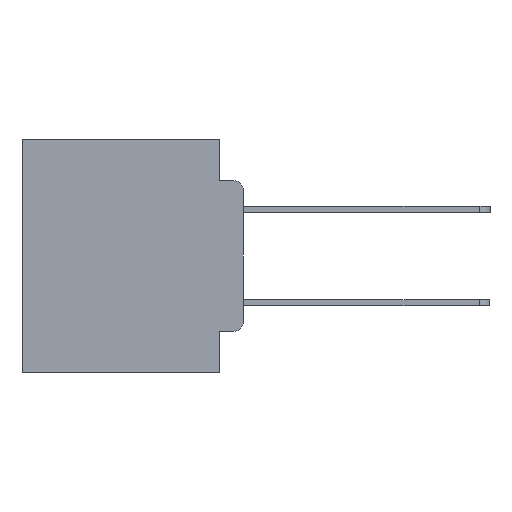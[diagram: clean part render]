
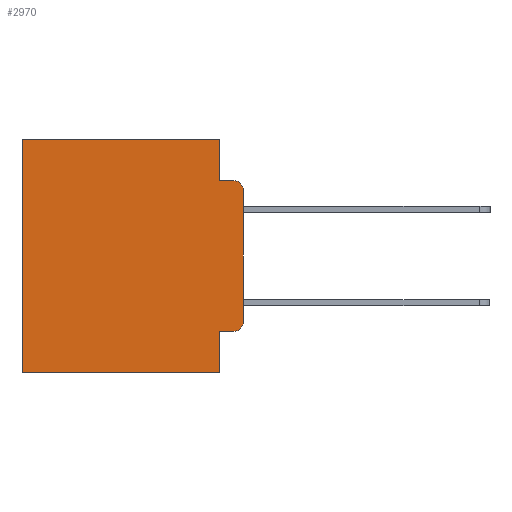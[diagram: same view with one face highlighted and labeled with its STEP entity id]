
A CAD part, left-side view. The second image highlights one B-rep face of the part: STEP entity #2970.
In plain terms, the highlighted planar face has unit normal (-1, 0, 0).
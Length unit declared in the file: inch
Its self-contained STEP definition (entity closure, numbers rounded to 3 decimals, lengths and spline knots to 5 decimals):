
#511 = EDGE_CURVE ( 'NONE', #17924, #20325, #26885, .T. ) ;
#786 = DIRECTION ( 'NONE',  ( 1., 0., 0. ) ) ;
#950 = EDGE_CURVE ( 'NONE', #10034, #12043, #11070, .T. ) ;
#1127 = DIRECTION ( 'NONE',  ( 0., 0., -1. ) ) ;
#1162 = CARTESIAN_POINT ( 'NONE',  ( 0.298, 0.051, -0.5 ) ) ;
#1786 = DIRECTION ( 'NONE',  ( 0., 0., -1. ) ) ;
#1940 = CARTESIAN_POINT ( 'NONE',  ( 0.298, 0.473, 0. ) ) ;
#2078 = CARTESIAN_POINT ( 'NONE',  ( 0.298, 0., 0. ) ) ;
#2630 = ORIENTED_EDGE ( 'NONE', *, *, #7078, .F. ) ;
#2756 = CARTESIAN_POINT ( 'NONE',  ( 0.298, 0.02, -0.0885 ) ) ;
#2970 = ADVANCED_FACE ( 'NONE', ( #5339 ), #6437, .F. ) ;
#3046 = VERTEX_POINT ( 'NONE', #18822 ) ;
#4294 = VERTEX_POINT ( 'NONE', #19255 ) ;
#4443 = DIRECTION ( 'NONE',  ( -1., 0., 0. ) ) ;
#4648 = DIRECTION ( 'NONE',  ( 0., -1., 0. ) ) ;
#4677 = EDGE_CURVE ( 'NONE', #3046, #8302, #20778, .T. ) ;
#4717 = ORIENTED_EDGE ( 'NONE', *, *, #4677, .F. ) ;
#4980 = CIRCLE ( 'NONE', #23388, 0.02 ) ;
#5144 = DIRECTION ( 'NONE',  ( 0., 0., -1. ) ) ;
#5167 = CARTESIAN_POINT ( 'NONE',  ( 0.298, 0.051, -0.4115 ) ) ;
#5240 = ORIENTED_EDGE ( 'NONE', *, *, #21757, .T. ) ;
#5339 = FACE_OUTER_BOUND ( 'NONE', #23997, .T. ) ;
#6437 = PLANE ( 'NONE',  #23172 ) ;
#7078 = EDGE_CURVE ( 'NONE', #21156, #8940, #7230, .T. ) ;
#7223 = DIRECTION ( 'NONE',  ( 0., 0., -1. ) ) ;
#7230 = LINE ( 'NONE', #19972, #23930 ) ;
#8302 = VERTEX_POINT ( 'NONE', #9517 ) ;
#8361 = ORIENTED_EDGE ( 'NONE', *, *, #24589, .T. ) ;
#8940 = VERTEX_POINT ( 'NONE', #2756 ) ;
#9263 = ORIENTED_EDGE ( 'NONE', *, *, #10121, .T. ) ;
#9517 = CARTESIAN_POINT ( 'NONE',  ( 0.298, 0., -0.3915 ) ) ;
#10034 = VERTEX_POINT ( 'NONE', #19472 ) ;
#10121 = EDGE_CURVE ( 'NONE', #3046, #8940, #12650, .T. ) ;
#10365 = CARTESIAN_POINT ( 'NONE',  ( 0.298, 0., 0. ) ) ;
#10659 = DIRECTION ( 'NONE',  ( 0., 0., -1. ) ) ;
#10938 = VECTOR ( 'NONE', #10659, 39.37008 ) ;
#11070 = LINE ( 'NONE', #2078, #18244 ) ;
#11569 = VECTOR ( 'NONE', #7223, 39.37008 ) ;
#11845 = CARTESIAN_POINT ( 'NONE',  ( 0.298, 0.051, -0.0885 ) ) ;
#11899 = DIRECTION ( 'NONE',  ( 0., -1., 0. ) ) ;
#12043 = VERTEX_POINT ( 'NONE', #1940 ) ;
#12581 = ORIENTED_EDGE ( 'NONE', *, *, #18916, .F. ) ;
#12650 = CIRCLE ( 'NONE', #15626, 0.02 ) ;
#13063 = EDGE_CURVE ( 'NONE', #10034, #21156, #20383, .T. ) ;
#14457 = CARTESIAN_POINT ( 'NONE',  ( 0.298, 0.051, 0. ) ) ;
#14480 = DIRECTION ( 'NONE',  ( -1., 0., 0. ) ) ;
#14549 = DIRECTION ( 'NONE',  ( 0., 0., -1. ) ) ;
#14694 = ORIENTED_EDGE ( 'NONE', *, *, #950, .T. ) ;
#14816 = ORIENTED_EDGE ( 'NONE', *, *, #13063, .F. ) ;
#14891 = VECTOR ( 'NONE', #11899, 39.37008 ) ;
#14919 = VECTOR ( 'NONE', #25075, 39.37008 ) ;
#15027 = ORIENTED_EDGE ( 'NONE', *, *, #17442, .T. ) ;
#15201 = CARTESIAN_POINT ( 'NONE',  ( 0.298, 0.473, 0. ) ) ;
#15405 = CARTESIAN_POINT ( 'NONE',  ( 0.298, 0., -0.5 ) ) ;
#15626 = AXIS2_PLACEMENT_3D ( 'NONE', #17655, #4443, #19852 ) ;
#15870 = CARTESIAN_POINT ( 'NONE',  ( 0.298, 0.02, -0.4115 ) ) ;
#17442 = EDGE_CURVE ( 'NONE', #12043, #20325, #27381, .T. ) ;
#17655 = CARTESIAN_POINT ( 'NONE',  ( 0.298, 0.02, -0.1085 ) ) ;
#17924 = VERTEX_POINT ( 'NONE', #1162 ) ;
#18220 = CARTESIAN_POINT ( 'NONE',  ( 0.298, 0.051, 0. ) ) ;
#18244 = VECTOR ( 'NONE', #22523, 39.37008 ) ;
#18822 = CARTESIAN_POINT ( 'NONE',  ( 0.298, 0., -0.1085 ) ) ;
#18916 = EDGE_CURVE ( 'NONE', #4294, #17924, #27299, .T. ) ;
#19255 = CARTESIAN_POINT ( 'NONE',  ( 0.298, 0.051, -0.4115 ) ) ;
#19472 = CARTESIAN_POINT ( 'NONE',  ( 0.298, 0.051, 0. ) ) ;
#19852 = DIRECTION ( 'NONE',  ( 0., 0., -1. ) ) ;
#19972 = CARTESIAN_POINT ( 'NONE',  ( 0.298, 0.051, -0.0885 ) ) ;
#20325 = VERTEX_POINT ( 'NONE', #21547 ) ;
#20383 = LINE ( 'NONE', #14457, #25322 ) ;
#20559 = CARTESIAN_POINT ( 'NONE',  ( 0.298, 0., 0. ) ) ;
#20617 = LINE ( 'NONE', #5167, #14891 ) ;
#20778 = LINE ( 'NONE', #20559, #25705 ) ;
#21156 = VERTEX_POINT ( 'NONE', #11845 ) ;
#21547 = CARTESIAN_POINT ( 'NONE',  ( 0.298, 0.473, -0.5 ) ) ;
#21757 = EDGE_CURVE ( 'NONE', #4294, #25067, #20617, .T. ) ;
#22523 = DIRECTION ( 'NONE',  ( 0., 1., 0. ) ) ;
#23172 = AXIS2_PLACEMENT_3D ( 'NONE', #10365, #786, #1786 ) ;
#23388 = AXIS2_PLACEMENT_3D ( 'NONE', #27206, #14480, #1127 ) ;
#23930 = VECTOR ( 'NONE', #4648, 39.37008 ) ;
#23997 = EDGE_LOOP ( 'NONE', ( #4717, #9263, #2630, #14816, #14694, #15027, #26645, #12581, #5240, #8361 ) ) ;
#24589 = EDGE_CURVE ( 'NONE', #25067, #8302, #4980, .T. ) ;
#25067 = VERTEX_POINT ( 'NONE', #15870 ) ;
#25075 = DIRECTION ( 'NONE',  ( 0., 1., 0. ) ) ;
#25322 = VECTOR ( 'NONE', #14549, 39.37008 ) ;
#25705 = VECTOR ( 'NONE', #5144, 39.37008 ) ;
#26645 = ORIENTED_EDGE ( 'NONE', *, *, #511, .F. ) ;
#26885 = LINE ( 'NONE', #15405, #14919 ) ;
#27206 = CARTESIAN_POINT ( 'NONE',  ( 0.298, 0.02, -0.3915 ) ) ;
#27299 = LINE ( 'NONE', #18220, #11569 ) ;
#27381 = LINE ( 'NONE', #15201, #10938 ) ;
